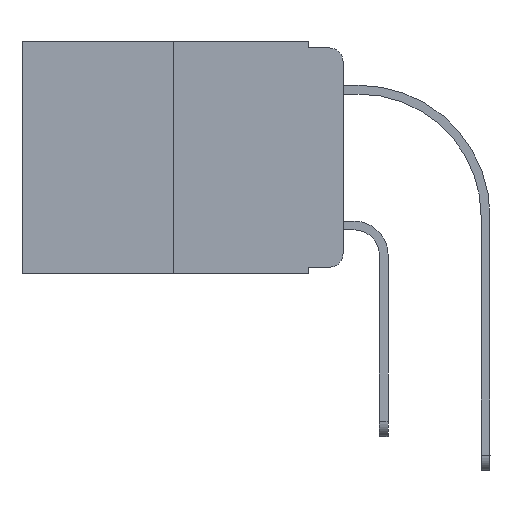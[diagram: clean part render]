
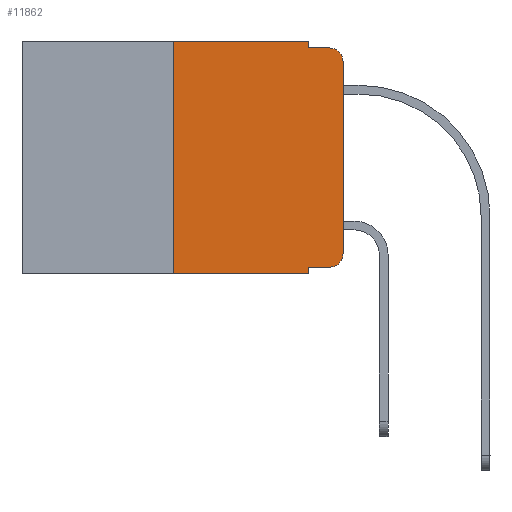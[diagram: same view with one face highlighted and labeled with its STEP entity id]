
A CAD part, left-side view. The second image highlights one B-rep face of the part: STEP entity #11862.
In plain terms, the highlighted planar face has unit normal (-1, 0, 0).
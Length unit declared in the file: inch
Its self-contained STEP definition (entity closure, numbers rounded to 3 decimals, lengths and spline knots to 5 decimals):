
#1062 = LINE ( 'NONE', #18990, #21322 ) ;
#1139 = ORIENTED_EDGE ( 'NONE', *, *, #25619, .T. ) ;
#1162 = CARTESIAN_POINT ( 'NONE',  ( 0., 0.02, -0.03 ) ) ;
#1343 = VECTOR ( 'NONE', #4477, 39.37008 ) ;
#1632 = ORIENTED_EDGE ( 'NONE', *, *, #4050, .T. ) ;
#2645 = DIRECTION ( 'NONE',  ( -1., 0., 0. ) ) ;
#3966 = VECTOR ( 'NONE', #20699, 39.37008 ) ;
#4050 = EDGE_CURVE ( 'NONE', #15847, #16525, #5378, .T. ) ;
#4057 = CARTESIAN_POINT ( 'NONE',  ( 0., 0.051, -0.333 ) ) ;
#4076 = ORIENTED_EDGE ( 'NONE', *, *, #23180, .F. ) ;
#4267 = CARTESIAN_POINT ( 'NONE',  ( 0., 0.051, -0.01 ) ) ;
#4477 = DIRECTION ( 'NONE',  ( 0., 0., -1. ) ) ;
#4529 = DIRECTION ( 'NONE',  ( 0., -1., 0. ) ) ;
#4534 = LINE ( 'NONE', #4267, #11930 ) ;
#5163 = PLANE ( 'NONE',  #20160 ) ;
#5301 = FACE_OUTER_BOUND ( 'NONE', #5916, .T. ) ;
#5378 = CIRCLE ( 'NONE', #8753, 0.02 ) ;
#5779 = DIRECTION ( 'NONE',  ( 0., -1., 0. ) ) ;
#5916 = EDGE_LOOP ( 'NONE', ( #6711, #21683, #21685, #25145, #4076, #7601, #9731, #11853, #1139, #1632 ) ) ;
#6711 = ORIENTED_EDGE ( 'NONE', *, *, #21816, .T. ) ;
#7055 = VERTEX_POINT ( 'NONE', #9678 ) ;
#7163 = CARTESIAN_POINT ( 'NONE',  ( 0., 0.02, -0.01 ) ) ;
#7387 = VERTEX_POINT ( 'NONE', #13230 ) ;
#7601 = ORIENTED_EDGE ( 'NONE', *, *, #20231, .F. ) ;
#7630 = LINE ( 'NONE', #7891, #25733 ) ;
#7669 = DIRECTION ( 'NONE',  ( 0., 0., -1. ) ) ;
#7891 = CARTESIAN_POINT ( 'NONE',  ( 0., 0.051, -0.333 ) ) ;
#8657 = EDGE_CURVE ( 'NONE', #14988, #7055, #10583, .T. ) ;
#8753 = AXIS2_PLACEMENT_3D ( 'NONE', #13265, #2645, #14731 ) ;
#8915 = VERTEX_POINT ( 'NONE', #16275 ) ;
#9008 = VERTEX_POINT ( 'NONE', #10037 ) ;
#9117 = DIRECTION ( 'NONE',  ( 0., 0., -1. ) ) ;
#9678 = CARTESIAN_POINT ( 'NONE',  ( 0., 0.051, -0.343 ) ) ;
#9731 = ORIENTED_EDGE ( 'NONE', *, *, #13961, .T. ) ;
#10037 = CARTESIAN_POINT ( 'NONE',  ( 0., 0.051, 0. ) ) ;
#10063 = CIRCLE ( 'NONE', #24889, 0.02 ) ;
#10583 = LINE ( 'NONE', #22810, #1343 ) ;
#10718 = CARTESIAN_POINT ( 'NONE',  ( 0., 0., -0.03 ) ) ;
#11260 = CARTESIAN_POINT ( 'NONE',  ( 0., 0.473, 0. ) ) ;
#11523 = DIRECTION ( 'NONE',  ( 0., 0., -1. ) ) ;
#11853 = ORIENTED_EDGE ( 'NONE', *, *, #8657, .F. ) ;
#11862 = ADVANCED_FACE ( 'NONE', ( #5301 ), #5163, .F. ) ;
#11930 = VECTOR ( 'NONE', #5779, 39.37008 ) ;
#13230 = CARTESIAN_POINT ( 'NONE',  ( 0., 0.25, -0.343 ) ) ;
#13265 = CARTESIAN_POINT ( 'NONE',  ( 0., 0.02, -0.313 ) ) ;
#13961 = EDGE_CURVE ( 'NONE', #7387, #7055, #19565, .T. ) ;
#14571 = CARTESIAN_POINT ( 'NONE',  ( 0., 0., 0. ) ) ;
#14731 = DIRECTION ( 'NONE',  ( 0., 0., -1. ) ) ;
#14867 = EDGE_CURVE ( 'NONE', #23442, #19085, #10063, .T. ) ;
#14988 = VERTEX_POINT ( 'NONE', #4057 ) ;
#15341 = VERTEX_POINT ( 'NONE', #16358 ) ;
#15455 = CARTESIAN_POINT ( 'NONE',  ( 0., 0.473, -0.343 ) ) ;
#15847 = VERTEX_POINT ( 'NONE', #25786 ) ;
#16275 = CARTESIAN_POINT ( 'NONE',  ( 0., 0.051, -0.01 ) ) ;
#16358 = CARTESIAN_POINT ( 'NONE',  ( 0., 0.25, 0. ) ) ;
#16384 = VECTOR ( 'NONE', #23031, 39.37008 ) ;
#16525 = VERTEX_POINT ( 'NONE', #24536 ) ;
#18009 = EDGE_CURVE ( 'NONE', #9008, #8915, #19352, .T. ) ;
#18078 = VECTOR ( 'NONE', #4529, 39.37008 ) ;
#18323 = EDGE_CURVE ( 'NONE', #8915, #19085, #4534, .T. ) ;
#18990 = CARTESIAN_POINT ( 'NONE',  ( 0., 0.25, 0. ) ) ;
#19000 = LINE ( 'NONE', #22718, #18078 ) ;
#19085 = VERTEX_POINT ( 'NONE', #7163 ) ;
#19352 = LINE ( 'NONE', #23868, #20376 ) ;
#19565 = LINE ( 'NONE', #15455, #16384 ) ;
#20160 = AXIS2_PLACEMENT_3D ( 'NONE', #11260, #23223, #11523 ) ;
#20231 = EDGE_CURVE ( 'NONE', #7387, #15341, #1062, .T. ) ;
#20376 = VECTOR ( 'NONE', #7669, 39.37008 ) ;
#20699 = DIRECTION ( 'NONE',  ( 0., 0., 1. ) ) ;
#21322 = VECTOR ( 'NONE', #23365, 39.37008 ) ;
#21683 = ORIENTED_EDGE ( 'NONE', *, *, #14867, .T. ) ;
#21685 = ORIENTED_EDGE ( 'NONE', *, *, #18323, .F. ) ;
#21816 = EDGE_CURVE ( 'NONE', #16525, #23442, #24657, .T. ) ;
#22718 = CARTESIAN_POINT ( 'NONE',  ( 0., 0.473, 0. ) ) ;
#22810 = CARTESIAN_POINT ( 'NONE',  ( 0., 0.051, 0. ) ) ;
#23031 = DIRECTION ( 'NONE',  ( 0., -1., 0. ) ) ;
#23180 = EDGE_CURVE ( 'NONE', #15341, #9008, #19000, .T. ) ;
#23223 = DIRECTION ( 'NONE',  ( 1., 0., 0. ) ) ;
#23365 = DIRECTION ( 'NONE',  ( 0., 0., 1. ) ) ;
#23442 = VERTEX_POINT ( 'NONE', #10718 ) ;
#23702 = DIRECTION ( 'NONE',  ( 0., -1., 0. ) ) ;
#23727 = DIRECTION ( 'NONE',  ( -1., 0., 0. ) ) ;
#23868 = CARTESIAN_POINT ( 'NONE',  ( 0., 0.051, 0. ) ) ;
#24536 = CARTESIAN_POINT ( 'NONE',  ( 0., 0., -0.313 ) ) ;
#24657 = LINE ( 'NONE', #14571, #3966 ) ;
#24889 = AXIS2_PLACEMENT_3D ( 'NONE', #1162, #23727, #9117 ) ;
#25145 = ORIENTED_EDGE ( 'NONE', *, *, #18009, .F. ) ;
#25619 = EDGE_CURVE ( 'NONE', #14988, #15847, #7630, .T. ) ;
#25733 = VECTOR ( 'NONE', #23702, 39.37008 ) ;
#25786 = CARTESIAN_POINT ( 'NONE',  ( 0., 0.02, -0.333 ) ) ;
